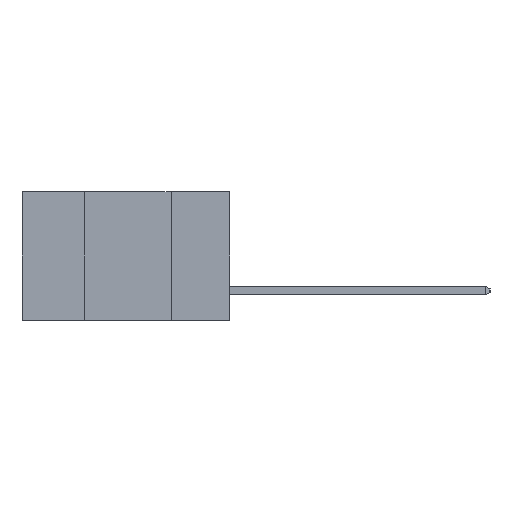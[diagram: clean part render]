
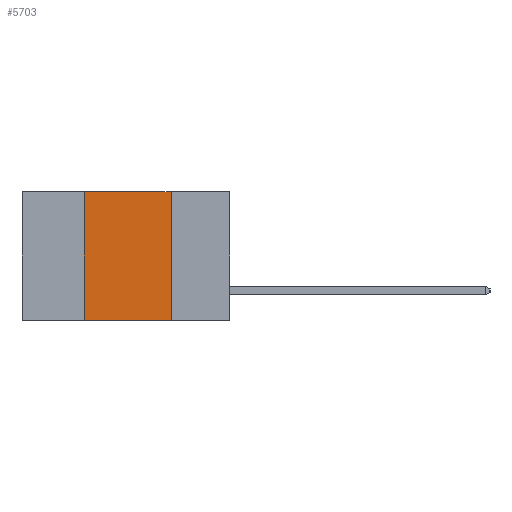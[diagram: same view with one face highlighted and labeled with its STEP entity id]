
A CAD part, left-side view. The second image highlights one B-rep face of the part: STEP entity #5703.
In plain terms, the highlighted planar face has unit normal (-1, 0, 0).
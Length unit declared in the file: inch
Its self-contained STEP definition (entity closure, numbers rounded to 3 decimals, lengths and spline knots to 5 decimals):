
#252 = PLANE ( 'NONE',  #9118 ) ;
#455 = CARTESIAN_POINT ( 'NONE',  ( 0., 0.42, 0. ) ) ;
#1072 = EDGE_CURVE ( 'NONE', #7973, #2888, #1864, .T. ) ;
#1301 = DIRECTION ( 'NONE',  ( 0., 0., -1. ) ) ;
#1378 = CARTESIAN_POINT ( 'NONE',  ( 0., 0.6, -0.37 ) ) ;
#1864 = LINE ( 'NONE', #455, #4326 ) ;
#2372 = ORIENTED_EDGE ( 'NONE', *, *, #1072, .F. ) ;
#2392 = CARTESIAN_POINT ( 'NONE',  ( 0., 0.17, -0.37 ) ) ;
#2888 = VERTEX_POINT ( 'NONE', #8315 ) ;
#4004 = LINE ( 'NONE', #10476, #11160 ) ;
#4151 = DIRECTION ( 'NONE',  ( 0., 0., -1. ) ) ;
#4326 = VECTOR ( 'NONE', #10616, 39.37008 ) ;
#4806 = ORIENTED_EDGE ( 'NONE', *, *, #7631, .F. ) ;
#5247 = LINE ( 'NONE', #8080, #7557 ) ;
#5420 = CARTESIAN_POINT ( 'NONE',  ( 0., 0.6, 0. ) ) ;
#5536 = LINE ( 'NONE', #1378, #11280 ) ;
#5703 = ADVANCED_FACE ( 'NONE', ( #8678 ), #252, .F. ) ;
#5726 = EDGE_LOOP ( 'NONE', ( #4806, #12571, #2372, #7744 ) ) ;
#5856 = CARTESIAN_POINT ( 'NONE',  ( 0., 0.42, -0.37 ) ) ;
#7320 = EDGE_CURVE ( 'NONE', #2888, #8551, #4004, .T. ) ;
#7405 = DIRECTION ( 'NONE',  ( 1., 0., 0. ) ) ;
#7478 = DIRECTION ( 'NONE',  ( 0., -1., 0. ) ) ;
#7557 = VECTOR ( 'NONE', #4151, 39.37008 ) ;
#7631 = EDGE_CURVE ( 'NONE', #8551, #9573, #5247, .T. ) ;
#7744 = ORIENTED_EDGE ( 'NONE', *, *, #10258, .T. ) ;
#7973 = VERTEX_POINT ( 'NONE', #5856 ) ;
#8080 = CARTESIAN_POINT ( 'NONE',  ( 0., 0.17, 0. ) ) ;
#8315 = CARTESIAN_POINT ( 'NONE',  ( 0., 0.42, 0. ) ) ;
#8551 = VERTEX_POINT ( 'NONE', #10571 ) ;
#8565 = DIRECTION ( 'NONE',  ( 0., -1., 0. ) ) ;
#8678 = FACE_OUTER_BOUND ( 'NONE', #5726, .T. ) ;
#9118 = AXIS2_PLACEMENT_3D ( 'NONE', #5420, #7405, #1301 ) ;
#9573 = VERTEX_POINT ( 'NONE', #2392 ) ;
#10258 = EDGE_CURVE ( 'NONE', #7973, #9573, #5536, .T. ) ;
#10476 = CARTESIAN_POINT ( 'NONE',  ( 0., 0.6, 0. ) ) ;
#10571 = CARTESIAN_POINT ( 'NONE',  ( 0., 0.17, 0. ) ) ;
#10616 = DIRECTION ( 'NONE',  ( 0., 0., 1. ) ) ;
#11160 = VECTOR ( 'NONE', #8565, 39.37008 ) ;
#11280 = VECTOR ( 'NONE', #7478, 39.37008 ) ;
#12571 = ORIENTED_EDGE ( 'NONE', *, *, #7320, .F. ) ;
